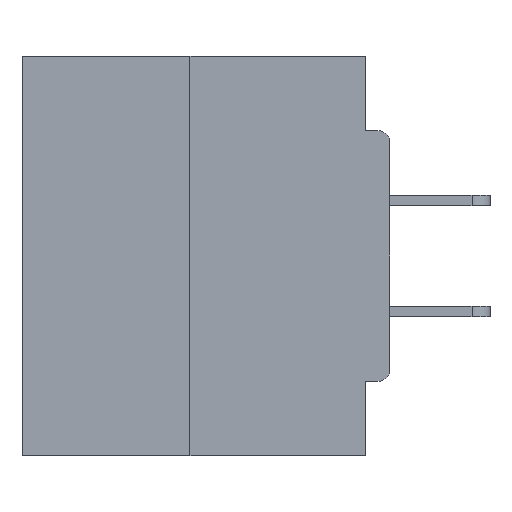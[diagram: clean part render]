
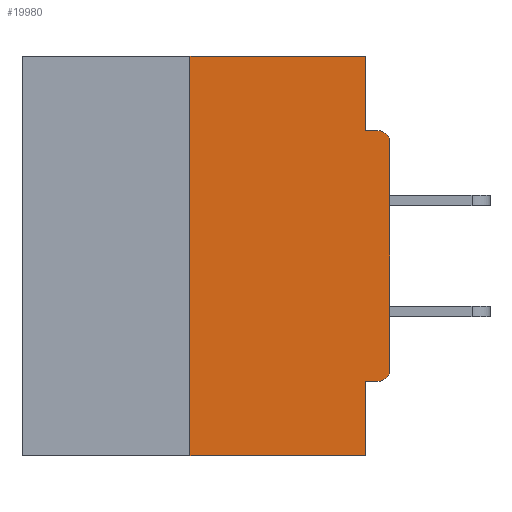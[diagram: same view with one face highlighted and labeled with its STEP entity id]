
A CAD part, left-side view. The second image highlights one B-rep face of the part: STEP entity #19980.
In plain terms, the highlighted planar face has unit normal (-1, 0, 0).
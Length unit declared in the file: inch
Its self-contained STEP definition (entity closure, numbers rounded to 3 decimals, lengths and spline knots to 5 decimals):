
#337 = FACE_OUTER_BOUND ( 'NONE', #23319, .T. ) ;
#650 = LINE ( 'NONE', #33217, #2722 ) ;
#2011 = LINE ( 'NONE', #14011, #12468 ) ;
#2654 = CARTESIAN_POINT ( 'NONE',  ( 0., 0.015, -0.3915 ) ) ;
#2722 = VECTOR ( 'NONE', #22167, 39.37008 ) ;
#2811 = ORIENTED_EDGE ( 'NONE', *, *, #14264, .F. ) ;
#2868 = DIRECTION ( 'NONE',  ( 0., 0., -1. ) ) ;
#2880 = CARTESIAN_POINT ( 'NONE',  ( 0., 0.46, 0. ) ) ;
#3786 = VECTOR ( 'NONE', #17279, 39.37008 ) ;
#3824 = DIRECTION ( 'NONE',  ( 0., 0., -1. ) ) ;
#3852 = EDGE_CURVE ( 'NONE', #6678, #32557, #10402, .T. ) ;
#4254 = CARTESIAN_POINT ( 'NONE',  ( 0., 0., -0.1085 ) ) ;
#5058 = LINE ( 'NONE', #2880, #23942 ) ;
#5558 = EDGE_CURVE ( 'NONE', #32557, #8782, #13275, .T. ) ;
#5605 = EDGE_CURVE ( 'NONE', #11496, #32761, #2011, .T. ) ;
#5808 = CARTESIAN_POINT ( 'NONE',  ( 0., 0., 0. ) ) ;
#5875 = EDGE_CURVE ( 'NONE', #10357, #33550, #15016, .T. ) ;
#6442 = CARTESIAN_POINT ( 'NONE',  ( 0., 0.031, -0.0935 ) ) ;
#6678 = VERTEX_POINT ( 'NONE', #23847 ) ;
#6686 = EDGE_CURVE ( 'NONE', #29810, #33241, #30919, .T. ) ;
#6869 = CARTESIAN_POINT ( 'NONE',  ( 0., 0.25, -0.5 ) ) ;
#7124 = VECTOR ( 'NONE', #15403, 39.37008 ) ;
#8782 = VERTEX_POINT ( 'NONE', #4254 ) ;
#9328 = DIRECTION ( 'NONE',  ( -1., 0., 0. ) ) ;
#9337 = DIRECTION ( 'NONE',  ( 1., 0., 0. ) ) ;
#9942 = EDGE_CURVE ( 'NONE', #6678, #11496, #13411, .T. ) ;
#10015 = CARTESIAN_POINT ( 'NONE',  ( 0., 0.015, -0.0935 ) ) ;
#10357 = VERTEX_POINT ( 'NONE', #6869 ) ;
#10402 = CIRCLE ( 'NONE', #24499, 0.015 ) ;
#10583 = ORIENTED_EDGE ( 'NONE', *, *, #12284, .F. ) ;
#11283 = DIRECTION ( 'NONE',  ( 0., 0., -1. ) ) ;
#11496 = VERTEX_POINT ( 'NONE', #17836 ) ;
#12178 = CIRCLE ( 'NONE', #16394, 0.015 ) ;
#12284 = EDGE_CURVE ( 'NONE', #33241, #30734, #650, .T. ) ;
#12468 = VECTOR ( 'NONE', #11283, 39.37008 ) ;
#12672 = DIRECTION ( 'NONE',  ( -1., 0., 0. ) ) ;
#12804 = CARTESIAN_POINT ( 'NONE',  ( 0., 0., -0.4065 ) ) ;
#12813 = VECTOR ( 'NONE', #2868, 39.37008 ) ;
#13275 = LINE ( 'NONE', #5808, #24154 ) ;
#13411 = LINE ( 'NONE', #12804, #7124 ) ;
#13520 = CARTESIAN_POINT ( 'NONE',  ( 0., 0.031, 0. ) ) ;
#14011 = CARTESIAN_POINT ( 'NONE',  ( 0., 0.031, -0.5 ) ) ;
#14262 = CARTESIAN_POINT ( 'NONE',  ( 0., 0.031, -0.5 ) ) ;
#14264 = EDGE_CURVE ( 'NONE', #33550, #29810, #5058, .T. ) ;
#14668 = CARTESIAN_POINT ( 'NONE',  ( 0., 0.46, -0.5 ) ) ;
#15016 = LINE ( 'NONE', #18686, #21343 ) ;
#15403 = DIRECTION ( 'NONE',  ( 0., 1., 0. ) ) ;
#16378 = CARTESIAN_POINT ( 'NONE',  ( 0., 0.031, 0. ) ) ;
#16394 = AXIS2_PLACEMENT_3D ( 'NONE', #28470, #12672, #31511 ) ;
#16584 = DIRECTION ( 'NONE',  ( 0., 0., 1. ) ) ;
#17279 = DIRECTION ( 'NONE',  ( 0., -1., 0. ) ) ;
#17324 = CARTESIAN_POINT ( 'NONE',  ( 0., 0.46, 0. ) ) ;
#17836 = CARTESIAN_POINT ( 'NONE',  ( 0., 0.031, -0.4065 ) ) ;
#18686 = CARTESIAN_POINT ( 'NONE',  ( 0., 0.25, 0. ) ) ;
#18946 = ORIENTED_EDGE ( 'NONE', *, *, #25913, .T. ) ;
#19104 = ORIENTED_EDGE ( 'NONE', *, *, #5605, .F. ) ;
#19325 = ORIENTED_EDGE ( 'NONE', *, *, #5558, .T. ) ;
#19980 = ADVANCED_FACE ( 'NONE', ( #337 ), #28259, .F. ) ;
#21343 = VECTOR ( 'NONE', #16584, 39.37008 ) ;
#21345 = CARTESIAN_POINT ( 'NONE',  ( 0., 0.25, 0. ) ) ;
#22167 = DIRECTION ( 'NONE',  ( 0., -1., 0. ) ) ;
#22964 = ORIENTED_EDGE ( 'NONE', *, *, #6686, .F. ) ;
#23319 = EDGE_LOOP ( 'NONE', ( #2811, #27205, #25084, #19104, #31947, #31880, #19325, #18946, #10583, #22964 ) ) ;
#23847 = CARTESIAN_POINT ( 'NONE',  ( 0., 0.015, -0.4065 ) ) ;
#23942 = VECTOR ( 'NONE', #32806, 39.37008 ) ;
#24154 = VECTOR ( 'NONE', #32576, 39.37008 ) ;
#24499 = AXIS2_PLACEMENT_3D ( 'NONE', #2654, #9328, #3824 ) ;
#25084 = ORIENTED_EDGE ( 'NONE', *, *, #31719, .T. ) ;
#25205 = LINE ( 'NONE', #14668, #3786 ) ;
#25913 = EDGE_CURVE ( 'NONE', #8782, #30734, #12178, .T. ) ;
#27205 = ORIENTED_EDGE ( 'NONE', *, *, #5875, .F. ) ;
#27968 = AXIS2_PLACEMENT_3D ( 'NONE', #17324, #9337, #30612 ) ;
#28182 = CARTESIAN_POINT ( 'NONE',  ( 0., 0., -0.3915 ) ) ;
#28259 = PLANE ( 'NONE',  #27968 ) ;
#28470 = CARTESIAN_POINT ( 'NONE',  ( 0., 0.015, -0.1085 ) ) ;
#29810 = VERTEX_POINT ( 'NONE', #16378 ) ;
#30612 = DIRECTION ( 'NONE',  ( 0., 0., -1. ) ) ;
#30734 = VERTEX_POINT ( 'NONE', #10015 ) ;
#30919 = LINE ( 'NONE', #13520, #12813 ) ;
#31511 = DIRECTION ( 'NONE',  ( 0., 0., -1. ) ) ;
#31719 = EDGE_CURVE ( 'NONE', #10357, #32761, #25205, .T. ) ;
#31880 = ORIENTED_EDGE ( 'NONE', *, *, #3852, .T. ) ;
#31947 = ORIENTED_EDGE ( 'NONE', *, *, #9942, .F. ) ;
#32557 = VERTEX_POINT ( 'NONE', #28182 ) ;
#32576 = DIRECTION ( 'NONE',  ( 0., 0., 1. ) ) ;
#32761 = VERTEX_POINT ( 'NONE', #14262 ) ;
#32806 = DIRECTION ( 'NONE',  ( 0., -1., 0. ) ) ;
#33217 = CARTESIAN_POINT ( 'NONE',  ( 0., 0., -0.0935 ) ) ;
#33241 = VERTEX_POINT ( 'NONE', #6442 ) ;
#33550 = VERTEX_POINT ( 'NONE', #21345 ) ;
